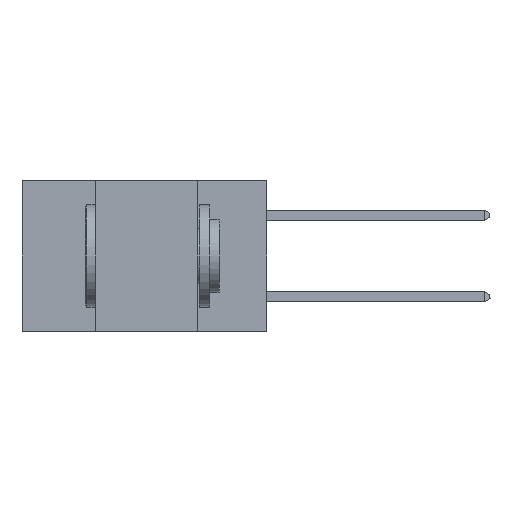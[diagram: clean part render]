
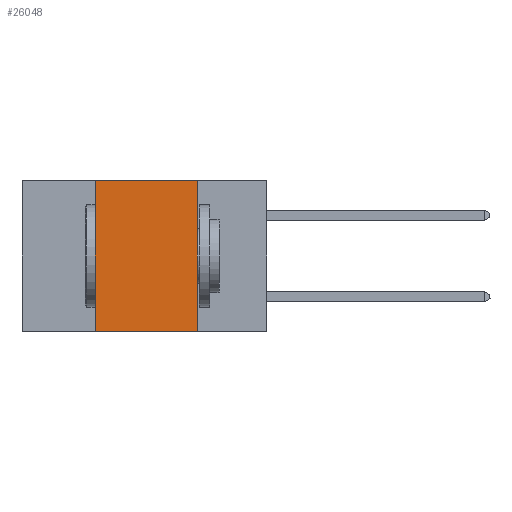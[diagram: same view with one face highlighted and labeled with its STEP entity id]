
A CAD part, left-side view. The second image highlights one B-rep face of the part: STEP entity #26048.
In plain terms, the highlighted planar face has unit normal (-1, 0, 0).
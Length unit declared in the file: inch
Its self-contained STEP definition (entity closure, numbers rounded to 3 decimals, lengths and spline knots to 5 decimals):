
#69 = LINE ( 'NONE', #27850, #23916 ) ;
#1407 = ORIENTED_EDGE ( 'NONE', *, *, #15563, .F. ) ;
#1414 = VECTOR ( 'NONE', #25868, 39.37008 ) ;
#3734 = CARTESIAN_POINT ( 'NONE',  ( 0., 0.6, 0. ) ) ;
#3775 = CARTESIAN_POINT ( 'NONE',  ( 0., 0.42, -0.37 ) ) ;
#4372 = EDGE_LOOP ( 'NONE', ( #1407, #9658, #15241, #22163 ) ) ;
#4520 = LINE ( 'NONE', #11238, #1414 ) ;
#5689 = DIRECTION ( 'NONE',  ( 0., 0., -1. ) ) ;
#7724 = VECTOR ( 'NONE', #20762, 39.37008 ) ;
#9658 = ORIENTED_EDGE ( 'NONE', *, *, #11804, .F. ) ;
#11027 = DIRECTION ( 'NONE',  ( 0., -1., 0. ) ) ;
#11238 = CARTESIAN_POINT ( 'NONE',  ( 0., 0.42, 0. ) ) ;
#11804 = EDGE_CURVE ( 'NONE', #30846, #26670, #31123, .T. ) ;
#12882 = PLANE ( 'NONE',  #16232 ) ;
#13093 = DIRECTION ( 'NONE',  ( 0., -1., 0. ) ) ;
#15241 = ORIENTED_EDGE ( 'NONE', *, *, #23860, .F. ) ;
#15374 = DIRECTION ( 'NONE',  ( 1., 0., 0. ) ) ;
#15416 = LINE ( 'NONE', #20971, #7724 ) ;
#15563 = EDGE_CURVE ( 'NONE', #26670, #31094, #15416, .T. ) ;
#15757 = CARTESIAN_POINT ( 'NONE',  ( 0., 0.17, -0.37 ) ) ;
#16232 = AXIS2_PLACEMENT_3D ( 'NONE', #18166, #15374, #5689 ) ;
#18166 = CARTESIAN_POINT ( 'NONE',  ( 0., 0.6, 0. ) ) ;
#19528 = CARTESIAN_POINT ( 'NONE',  ( 0., 0.42, 0. ) ) ;
#20332 = VERTEX_POINT ( 'NONE', #3775 ) ;
#20762 = DIRECTION ( 'NONE',  ( 0., 0., -1. ) ) ;
#20971 = CARTESIAN_POINT ( 'NONE',  ( 0., 0.17, 0. ) ) ;
#22163 = ORIENTED_EDGE ( 'NONE', *, *, #29126, .T. ) ;
#23490 = CARTESIAN_POINT ( 'NONE',  ( 0., 0.17, 0. ) ) ;
#23860 = EDGE_CURVE ( 'NONE', #20332, #30846, #4520, .T. ) ;
#23916 = VECTOR ( 'NONE', #13093, 39.37008 ) ;
#25868 = DIRECTION ( 'NONE',  ( 0., 0., 1. ) ) ;
#26048 = ADVANCED_FACE ( 'NONE', ( #28606 ), #12882, .F. ) ;
#26670 = VERTEX_POINT ( 'NONE', #23490 ) ;
#27850 = CARTESIAN_POINT ( 'NONE',  ( 0., 0.6, -0.37 ) ) ;
#28606 = FACE_OUTER_BOUND ( 'NONE', #4372, .T. ) ;
#29126 = EDGE_CURVE ( 'NONE', #20332, #31094, #69, .T. ) ;
#30846 = VERTEX_POINT ( 'NONE', #19528 ) ;
#31094 = VERTEX_POINT ( 'NONE', #15757 ) ;
#31123 = LINE ( 'NONE', #3734, #31512 ) ;
#31512 = VECTOR ( 'NONE', #11027, 39.37008 ) ;
